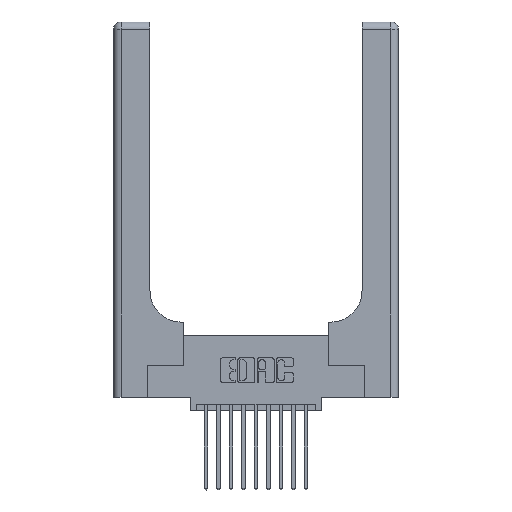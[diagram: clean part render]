
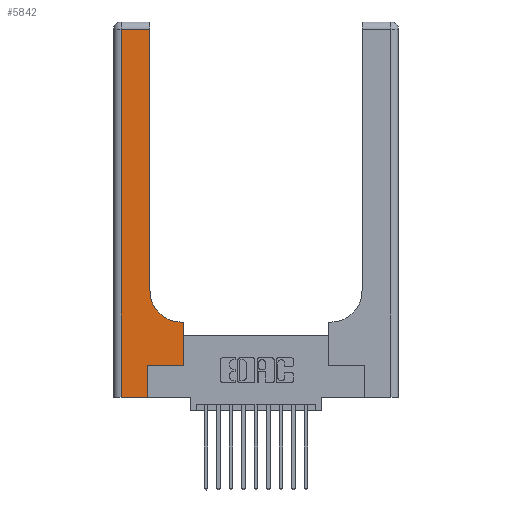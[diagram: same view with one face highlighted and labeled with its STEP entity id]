
A CAD part, top view. The second image highlights one B-rep face of the part: STEP entity #5842.
In plain terms, the highlighted planar face has unit normal (0, 0, 1).
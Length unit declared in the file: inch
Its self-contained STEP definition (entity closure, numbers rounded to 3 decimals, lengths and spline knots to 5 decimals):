
#813 = LINE ( 'NONE', #15095, #6530 ) ;
#1091 = CARTESIAN_POINT ( 'NONE',  ( 0.2915, 3., 0.37 ) ) ;
#1197 = LINE ( 'NONE', #6334, #7529 ) ;
#1746 = CIRCLE ( 'NONE', #11606, 0.25 ) ;
#1894 = EDGE_CURVE ( 'NONE', #3748, #11463, #7573, .T. ) ;
#2560 = EDGE_CURVE ( 'NONE', #12238, #3457, #813, .T. ) ;
#2616 = EDGE_LOOP ( 'NONE', ( #9525, #4482, #11147, #12678, #14017, #6228, #11165, #14389, #5149 ) ) ;
#3099 = EDGE_CURVE ( 'NONE', #4105, #15307, #7362, .T. ) ;
#3457 = VERTEX_POINT ( 'NONE', #11572 ) ;
#3552 = EDGE_CURVE ( 'NONE', #13760, #3748, #13626, .T. ) ;
#3584 = CARTESIAN_POINT ( 'NONE',  ( 0.5585, 0.25, 0.37 ) ) ;
#3652 = DIRECTION ( 'NONE',  ( 0., -1., 0. ) ) ;
#3748 = VERTEX_POINT ( 'NONE', #9206 ) ;
#4105 = VERTEX_POINT ( 'NONE', #8088 ) ;
#4482 = ORIENTED_EDGE ( 'NONE', *, *, #1894, .T. ) ;
#5149 = ORIENTED_EDGE ( 'NONE', *, *, #5532, .T. ) ;
#5265 = DIRECTION ( 'NONE',  ( 0., 1., 0. ) ) ;
#5385 = LINE ( 'NONE', #7494, #13300 ) ;
#5532 = EDGE_CURVE ( 'NONE', #3457, #13760, #1746, .T. ) ;
#5842 = ADVANCED_FACE ( 'NONE', ( #14336 ), #5937, .F. ) ;
#5912 = LINE ( 'NONE', #10469, #16815 ) ;
#5937 = PLANE ( 'NONE',  #15065 ) ;
#6228 = ORIENTED_EDGE ( 'NONE', *, *, #6744, .T. ) ;
#6308 = DIRECTION ( 'NONE',  ( -1., 0., 0. ) ) ;
#6334 = CARTESIAN_POINT ( 'NONE',  ( 0.06, 3., 0.37 ) ) ;
#6530 = VECTOR ( 'NONE', #9755, 39.37008 ) ;
#6744 = EDGE_CURVE ( 'NONE', #15737, #16119, #5385, .T. ) ;
#7102 = LINE ( 'NONE', #13818, #7919 ) ;
#7241 = CARTESIAN_POINT ( 'NONE',  ( 0., 3., 0.37 ) ) ;
#7362 = LINE ( 'NONE', #14327, #10405 ) ;
#7376 = DIRECTION ( 'NONE',  ( 0., 1., 0. ) ) ;
#7494 = CARTESIAN_POINT ( 'NONE',  ( 0.269, 0.25, 0.37 ) ) ;
#7529 = VECTOR ( 'NONE', #3652, 39.37008 ) ;
#7573 = LINE ( 'NONE', #14934, #10223 ) ;
#7609 = DIRECTION ( 'NONE',  ( 0., 1., 0. ) ) ;
#7650 = CARTESIAN_POINT ( 'NONE',  ( 0.269, 0.25, 0.37 ) ) ;
#7742 = VECTOR ( 'NONE', #7609, 39.37008 ) ;
#7919 = VECTOR ( 'NONE', #7376, 39.37008 ) ;
#8088 = CARTESIAN_POINT ( 'NONE',  ( 0.06, 0., 0.37 ) ) ;
#8332 = DIRECTION ( 'NONE',  ( -1., 0., 0. ) ) ;
#8444 = DIRECTION ( 'NONE',  ( 0., 0., -1. ) ) ;
#9206 = CARTESIAN_POINT ( 'NONE',  ( 0.2915, 2.94, 0.37 ) ) ;
#9525 = ORIENTED_EDGE ( 'NONE', *, *, #3552, .T. ) ;
#9755 = DIRECTION ( 'NONE',  ( -1., 0., 0. ) ) ;
#10071 = DIRECTION ( 'NONE',  ( 1., 0., 0. ) ) ;
#10223 = VECTOR ( 'NONE', #8332, 39.37008 ) ;
#10405 = VECTOR ( 'NONE', #13210, 39.37008 ) ;
#10469 = CARTESIAN_POINT ( 'NONE',  ( 0.5585, 0.25, 0.37 ) ) ;
#11147 = ORIENTED_EDGE ( 'NONE', *, *, #13896, .T. ) ;
#11165 = ORIENTED_EDGE ( 'NONE', *, *, #15343, .T. ) ;
#11463 = VERTEX_POINT ( 'NONE', #15594 ) ;
#11572 = CARTESIAN_POINT ( 'NONE',  ( 0.5415, 0.6, 0.37 ) ) ;
#11606 = AXIS2_PLACEMENT_3D ( 'NONE', #16179, #8444, #14648 ) ;
#12238 = VERTEX_POINT ( 'NONE', #12760 ) ;
#12252 = CARTESIAN_POINT ( 'NONE',  ( 0.2915, 0.85, 0.37 ) ) ;
#12678 = ORIENTED_EDGE ( 'NONE', *, *, #3099, .T. ) ;
#12760 = CARTESIAN_POINT ( 'NONE',  ( 0.5585, 0.6, 0.37 ) ) ;
#13210 = DIRECTION ( 'NONE',  ( 1., 0., 0. ) ) ;
#13300 = VECTOR ( 'NONE', #10071, 39.37008 ) ;
#13626 = LINE ( 'NONE', #1091, #7742 ) ;
#13760 = VERTEX_POINT ( 'NONE', #12252 ) ;
#13818 = CARTESIAN_POINT ( 'NONE',  ( 0.269, 0., 0.37 ) ) ;
#13896 = EDGE_CURVE ( 'NONE', #11463, #4105, #1197, .T. ) ;
#14017 = ORIENTED_EDGE ( 'NONE', *, *, #15051, .T. ) ;
#14327 = CARTESIAN_POINT ( 'NONE',  ( 0., 0., 0.37 ) ) ;
#14336 = FACE_OUTER_BOUND ( 'NONE', #2616, .T. ) ;
#14389 = ORIENTED_EDGE ( 'NONE', *, *, #2560, .T. ) ;
#14648 = DIRECTION ( 'NONE',  ( 1., 0., 0. ) ) ;
#14934 = CARTESIAN_POINT ( 'NONE',  ( 0., 2.94, 0.37 ) ) ;
#15051 = EDGE_CURVE ( 'NONE', #15307, #15737, #7102, .T. ) ;
#15065 = AXIS2_PLACEMENT_3D ( 'NONE', #7241, #16297, #6308 ) ;
#15095 = CARTESIAN_POINT ( 'NONE',  ( 0.2915, 0.6, 0.37 ) ) ;
#15307 = VERTEX_POINT ( 'NONE', #16797 ) ;
#15343 = EDGE_CURVE ( 'NONE', #16119, #12238, #5912, .T. ) ;
#15594 = CARTESIAN_POINT ( 'NONE',  ( 0.06, 2.94, 0.37 ) ) ;
#15737 = VERTEX_POINT ( 'NONE', #7650 ) ;
#16119 = VERTEX_POINT ( 'NONE', #3584 ) ;
#16179 = CARTESIAN_POINT ( 'NONE',  ( 0.5415, 0.85, 0.37 ) ) ;
#16297 = DIRECTION ( 'NONE',  ( 0., 0., -1. ) ) ;
#16797 = CARTESIAN_POINT ( 'NONE',  ( 0.269, 0., 0.37 ) ) ;
#16815 = VECTOR ( 'NONE', #5265, 39.37008 ) ;
